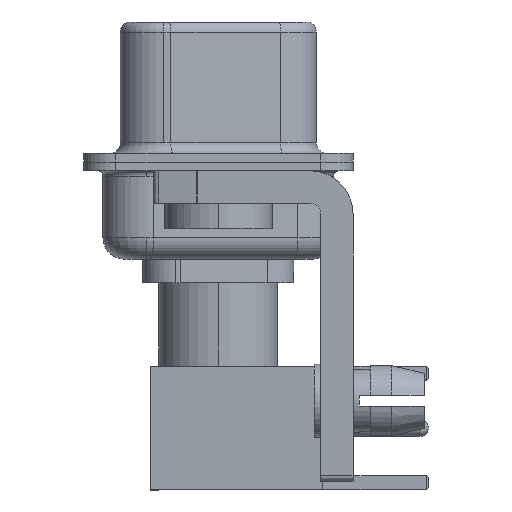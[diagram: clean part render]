
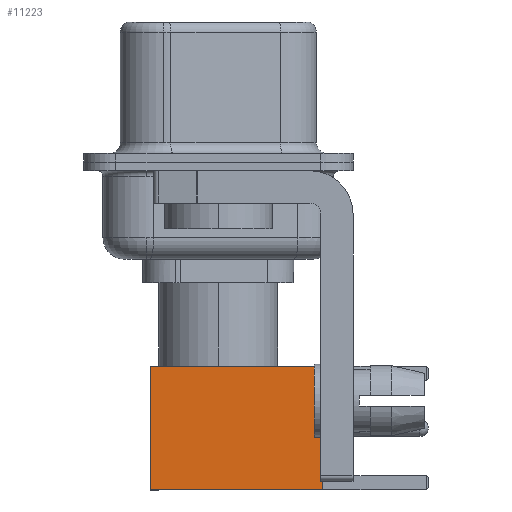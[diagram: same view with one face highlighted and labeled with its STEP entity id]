
A CAD part, left-side view. The second image highlights one B-rep face of the part: STEP entity #11223.
In plain terms, the highlighted face is planar.
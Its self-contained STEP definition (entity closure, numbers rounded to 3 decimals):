
#4 = VERTEX_POINT ( 'NONE', #11055 ) ;
#252 = CARTESIAN_POINT ( 'NONE',  ( -2.875, 2.875, 0. ) ) ;
#412 = DIRECTION ( 'NONE',  ( -1., 0., 0. ) ) ;
#607 = VECTOR ( 'NONE', #412, 1000. ) ;
#721 = ORIENTED_EDGE ( 'NONE', *, *, #6190, .T. ) ;
#1655 = CARTESIAN_POINT ( 'NONE',  ( 2.875, 2.875, 0. ) ) ;
#1742 = DIRECTION ( 'NONE',  ( 0., 0., -1. ) ) ;
#1802 = LINE ( 'NONE', #13196, #607 ) ;
#2263 = ORIENTED_EDGE ( 'NONE', *, *, #15898, .F. ) ;
#2748 = VERTEX_POINT ( 'NONE', #9756 ) ;
#3067 = VERTEX_POINT ( 'NONE', #13666 ) ;
#3143 = LINE ( 'NONE', #252, #15701 ) ;
#3898 = EDGE_CURVE ( 'NONE', #3067, #15484, #12790, .T. ) ;
#4325 = VECTOR ( 'NONE', #16889, 1000. ) ;
#5001 = EDGE_CURVE ( 'NONE', #4, #15484, #3143, .T. ) ;
#5942 = DIRECTION ( 'NONE',  ( 0., 0., -1. ) ) ;
#6190 = EDGE_CURVE ( 'NONE', #2748, #3067, #13230, .T. ) ;
#6966 = DIRECTION ( 'NONE',  ( 0., 0., 1. ) ) ;
#7152 = AXIS2_PLACEMENT_3D ( 'NONE', #18402, #15437, #6966 ) ;
#8184 = FACE_OUTER_BOUND ( 'NONE', #16759, .T. ) ;
#9721 = CARTESIAN_POINT ( 'NONE',  ( 0., 2.875, 0. ) ) ;
#9756 = CARTESIAN_POINT ( 'NONE',  ( 2.875, 2.875, 8. ) ) ;
#11030 = ORIENTED_EDGE ( 'NONE', *, *, #3898, .T. ) ;
#11055 = CARTESIAN_POINT ( 'NONE',  ( -2.875, 2.875, 8. ) ) ;
#11146 = PLANE ( 'NONE',  #7152 ) ;
#11223 = ADVANCED_FACE ( 'NONE', ( #8184 ), #11146, .T. ) ;
#11919 = ORIENTED_EDGE ( 'NONE', *, *, #5001, .F. ) ;
#12790 = LINE ( 'NONE', #9721, #4325 ) ;
#13196 = CARTESIAN_POINT ( 'NONE',  ( 0., 2.875, 8. ) ) ;
#13230 = LINE ( 'NONE', #1655, #17231 ) ;
#13666 = CARTESIAN_POINT ( 'NONE',  ( 2.875, 2.875, 0. ) ) ;
#15437 = DIRECTION ( 'NONE',  ( 0., 1., 0. ) ) ;
#15484 = VERTEX_POINT ( 'NONE', #17833 ) ;
#15701 = VECTOR ( 'NONE', #5942, 1000. ) ;
#15898 = EDGE_CURVE ( 'NONE', #2748, #4, #1802, .T. ) ;
#16759 = EDGE_LOOP ( 'NONE', ( #721, #11030, #11919, #2263 ) ) ;
#16889 = DIRECTION ( 'NONE',  ( -1., 0., 0. ) ) ;
#17231 = VECTOR ( 'NONE', #1742, 1000. ) ;
#17833 = CARTESIAN_POINT ( 'NONE',  ( -2.875, 2.875, 0. ) ) ;
#18402 = CARTESIAN_POINT ( 'NONE',  ( 2.875, 2.875, 0. ) ) ;
